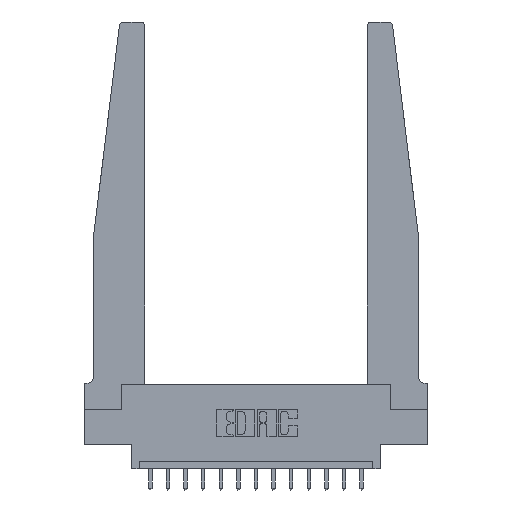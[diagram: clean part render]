
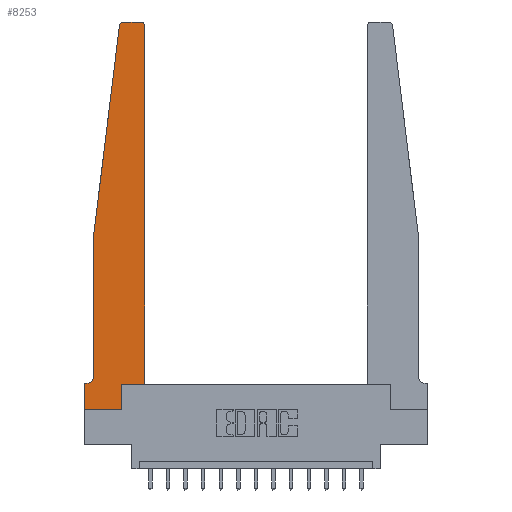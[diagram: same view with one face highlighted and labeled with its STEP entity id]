
A CAD part, top view. The second image highlights one B-rep face of the part: STEP entity #8253.
In plain terms, the highlighted planar face has unit normal (0, 0, 1).
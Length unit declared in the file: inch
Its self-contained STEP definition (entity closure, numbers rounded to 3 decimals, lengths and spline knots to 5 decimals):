
#111 = CARTESIAN_POINT ( 'NONE',  ( 0.2605, 0.18, 0.37 ) ) ;
#301 = AXIS2_PLACEMENT_3D ( 'NONE', #9756, #15086, #11331 ) ;
#533 = EDGE_CURVE ( 'NONE', #1208, #1429, #8440, .T. ) ;
#615 = LINE ( 'NONE', #958, #13233 ) ;
#728 = ORIENTED_EDGE ( 'NONE', *, *, #3240, .T. ) ;
#802 = VECTOR ( 'NONE', #11699, 39.37008 ) ;
#958 = CARTESIAN_POINT ( 'NONE',  ( 0.25, 2.75, 0.37 ) ) ;
#997 = CARTESIAN_POINT ( 'NONE',  ( 0.24675, 2.72367, 0.37 ) ) ;
#1208 = VERTEX_POINT ( 'NONE', #14766 ) ;
#1383 = ORIENTED_EDGE ( 'NONE', *, *, #12973, .T. ) ;
#1427 = CARTESIAN_POINT ( 'NONE',  ( 0.27653, 2.72, 0.37 ) ) ;
#1429 = VERTEX_POINT ( 'NONE', #5985 ) ;
#1726 = VERTEX_POINT ( 'NONE', #111 ) ;
#1769 = DIRECTION ( 'NONE',  ( 1., 0., 0. ) ) ;
#1774 = DIRECTION ( 'NONE',  ( 1., 0., 0. ) ) ;
#2218 = LINE ( 'NONE', #10040, #9789 ) ;
#2224 = ORIENTED_EDGE ( 'NONE', *, *, #533, .T. ) ;
#2546 = DIRECTION ( 'NONE',  ( 0., 1., 0. ) ) ;
#2828 = VERTEX_POINT ( 'NONE', #13530 ) ;
#2856 = DIRECTION ( 'NONE',  ( 0., -1., 0. ) ) ;
#2860 = EDGE_CURVE ( 'NONE', #1726, #5077, #4480, .T. ) ;
#2986 = EDGE_CURVE ( 'NONE', #10621, #15800, #13188, .T. ) ;
#3240 = EDGE_CURVE ( 'NONE', #5077, #10621, #5241, .T. ) ;
#4074 = CARTESIAN_POINT ( 'NONE',  ( 0.015, 0.2375, 0.37 ) ) ;
#4137 = ORIENTED_EDGE ( 'NONE', *, *, #5704, .T. ) ;
#4480 = LINE ( 'NONE', #13873, #11786 ) ;
#4518 = LINE ( 'NONE', #13475, #13294 ) ;
#5077 = VERTEX_POINT ( 'NONE', #15054 ) ;
#5241 = LINE ( 'NONE', #7735, #5303 ) ;
#5303 = VECTOR ( 'NONE', #2546, 39.37008 ) ;
#5461 = LINE ( 'NONE', #13727, #14972 ) ;
#5704 = EDGE_CURVE ( 'NONE', #15406, #6487, #2218, .T. ) ;
#5742 = CIRCLE ( 'NONE', #12733, 0.05 ) ;
#5985 = CARTESIAN_POINT ( 'NONE',  ( 0.2605, 0., 0.37 ) ) ;
#6110 = ORIENTED_EDGE ( 'NONE', *, *, #8869, .T. ) ;
#6487 = VERTEX_POINT ( 'NONE', #17277 ) ;
#6919 = FACE_OUTER_BOUND ( 'NONE', #16867, .T. ) ;
#7063 = ORIENTED_EDGE ( 'NONE', *, *, #8316, .T. ) ;
#7114 = CARTESIAN_POINT ( 'NONE',  ( 0.015, 0.1875, 0.37 ) ) ;
#7735 = CARTESIAN_POINT ( 'NONE',  ( 0.425, 0.18, 0.37 ) ) ;
#8064 = AXIS2_PLACEMENT_3D ( 'NONE', #1427, #16306, #16224 ) ;
#8215 = DIRECTION ( 'NONE',  ( 0., 0., -1. ) ) ;
#8253 = ADVANCED_FACE ( 'NONE', ( #6919 ), #13596, .T. ) ;
#8316 = EDGE_CURVE ( 'NONE', #15800, #11300, #615, .T. ) ;
#8440 = LINE ( 'NONE', #12805, #15986 ) ;
#8869 = EDGE_CURVE ( 'NONE', #15764, #11317, #9013, .T. ) ;
#8915 = CARTESIAN_POINT ( 'NONE',  ( 0.27653, 2.75, 0.37 ) ) ;
#9013 = LINE ( 'NONE', #14343, #14642 ) ;
#9736 = CARTESIAN_POINT ( 'NONE',  ( 0., 0.1875, 0.37 ) ) ;
#9756 = CARTESIAN_POINT ( 'NONE',  ( 0.395, 2.72, 0.37 ) ) ;
#9789 = VECTOR ( 'NONE', #9949, 39.37008 ) ;
#9949 = DIRECTION ( 'NONE',  ( -1., 0., 0. ) ) ;
#10040 = CARTESIAN_POINT ( 'NONE',  ( 0.065, 0.1875, 0.37 ) ) ;
#10621 = VERTEX_POINT ( 'NONE', #10695 ) ;
#10695 = CARTESIAN_POINT ( 'NONE',  ( 0.425, 2.72, 0.37 ) ) ;
#10759 = ORIENTED_EDGE ( 'NONE', *, *, #2860, .T. ) ;
#10975 = DIRECTION ( 'NONE',  ( 0., 0., 1. ) ) ;
#11300 = VERTEX_POINT ( 'NONE', #8915 ) ;
#11317 = VERTEX_POINT ( 'NONE', #16594 ) ;
#11331 = DIRECTION ( 'NONE',  ( 1., 0., 0. ) ) ;
#11682 = DIRECTION ( 'NONE',  ( -1., 0., 0. ) ) ;
#11699 = DIRECTION ( 'NONE',  ( 0., 1., 0. ) ) ;
#11786 = VECTOR ( 'NONE', #1774, 39.37008 ) ;
#11802 = ORIENTED_EDGE ( 'NONE', *, *, #2986, .T. ) ;
#12215 = ORIENTED_EDGE ( 'NONE', *, *, #15901, .T. ) ;
#12244 = DIRECTION ( 'NONE',  ( 0., -1., 0. ) ) ;
#12340 = ORIENTED_EDGE ( 'NONE', *, *, #16305, .T. ) ;
#12458 = EDGE_CURVE ( 'NONE', #6487, #1208, #4518, .T. ) ;
#12733 = AXIS2_PLACEMENT_3D ( 'NONE', #4074, #8215, #13457 ) ;
#12805 = CARTESIAN_POINT ( 'NONE',  ( 0., 0., 0.37 ) ) ;
#12896 = EDGE_CURVE ( 'NONE', #2828, #15406, #5742, .T. ) ;
#12973 = EDGE_CURVE ( 'NONE', #11317, #2828, #5461, .T. ) ;
#12987 = LINE ( 'NONE', #13080, #802 ) ;
#13080 = CARTESIAN_POINT ( 'NONE',  ( 0.2605, 0.18, 0.37 ) ) ;
#13188 = CIRCLE ( 'NONE', #301, 0.03 ) ;
#13233 = VECTOR ( 'NONE', #11682, 39.37008 ) ;
#13294 = VECTOR ( 'NONE', #2856, 39.37008 ) ;
#13378 = CIRCLE ( 'NONE', #8064, 0.03 ) ;
#13457 = DIRECTION ( 'NONE',  ( -1., 0., 0. ) ) ;
#13475 = CARTESIAN_POINT ( 'NONE',  ( 0., 0., 0.37 ) ) ;
#13530 = CARTESIAN_POINT ( 'NONE',  ( 0.065, 0.2375, 0.37 ) ) ;
#13596 = PLANE ( 'NONE',  #15741 ) ;
#13727 = CARTESIAN_POINT ( 'NONE',  ( 0.065, 1.25, 0.37 ) ) ;
#13873 = CARTESIAN_POINT ( 'NONE',  ( 0.425, 0.18, 0.37 ) ) ;
#14343 = CARTESIAN_POINT ( 'NONE',  ( 0.065, 1.25, 0.37 ) ) ;
#14642 = VECTOR ( 'NONE', #17049, 39.37008 ) ;
#14766 = CARTESIAN_POINT ( 'NONE',  ( 0., 0., 0.37 ) ) ;
#14972 = VECTOR ( 'NONE', #12244, 39.37008 ) ;
#15054 = CARTESIAN_POINT ( 'NONE',  ( 0.425, 0.18, 0.37 ) ) ;
#15086 = DIRECTION ( 'NONE',  ( 0., 0., 1. ) ) ;
#15151 = DIRECTION ( 'NONE',  ( 1., 0., 0. ) ) ;
#15406 = VERTEX_POINT ( 'NONE', #7114 ) ;
#15611 = ORIENTED_EDGE ( 'NONE', *, *, #12896, .T. ) ;
#15741 = AXIS2_PLACEMENT_3D ( 'NONE', #9736, #10975, #15151 ) ;
#15764 = VERTEX_POINT ( 'NONE', #997 ) ;
#15800 = VERTEX_POINT ( 'NONE', #15958 ) ;
#15901 = EDGE_CURVE ( 'NONE', #11300, #15764, #13378, .T. ) ;
#15948 = ORIENTED_EDGE ( 'NONE', *, *, #12458, .T. ) ;
#15958 = CARTESIAN_POINT ( 'NONE',  ( 0.395, 2.75, 0.37 ) ) ;
#15986 = VECTOR ( 'NONE', #1769, 39.37008 ) ;
#16224 = DIRECTION ( 'NONE',  ( 1., 0., 0. ) ) ;
#16305 = EDGE_CURVE ( 'NONE', #1429, #1726, #12987, .T. ) ;
#16306 = DIRECTION ( 'NONE',  ( 0., 0., 1. ) ) ;
#16594 = CARTESIAN_POINT ( 'NONE',  ( 0.065, 1.25, 0.37 ) ) ;
#16867 = EDGE_LOOP ( 'NONE', ( #7063, #12215, #6110, #1383, #15611, #4137, #15948, #2224, #12340, #10759, #728, #11802 ) ) ;
#17049 = DIRECTION ( 'NONE',  ( -0.122, -0.992, 0. ) ) ;
#17277 = CARTESIAN_POINT ( 'NONE',  ( 0., 0.1875, 0.37 ) ) ;
